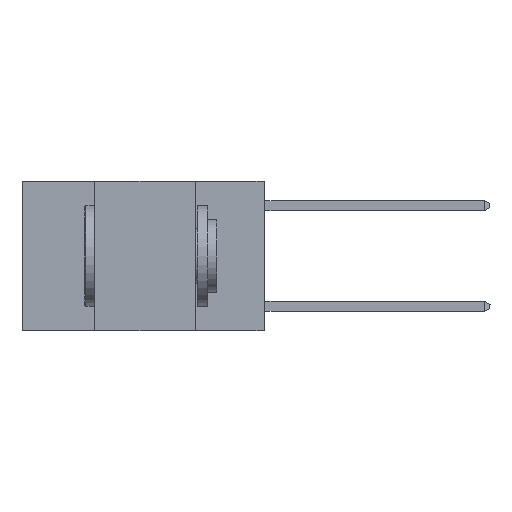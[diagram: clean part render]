
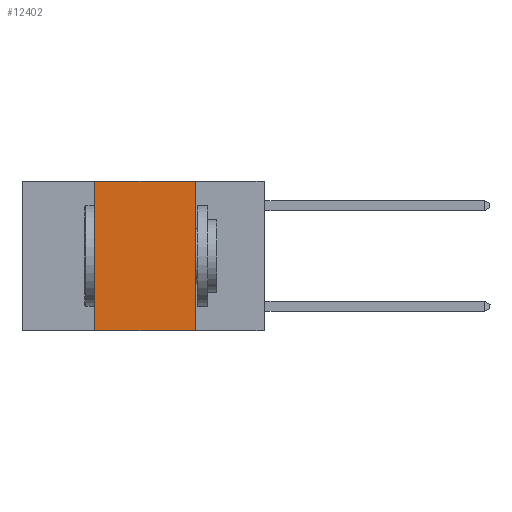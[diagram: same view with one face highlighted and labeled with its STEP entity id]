
A CAD part, left-side view. The second image highlights one B-rep face of the part: STEP entity #12402.
In plain terms, the highlighted planar face has unit normal (-1, 0, 0).
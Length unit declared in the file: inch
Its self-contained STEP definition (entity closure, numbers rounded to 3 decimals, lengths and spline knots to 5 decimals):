
#198 = PLANE ( 'NONE',  #18659 ) ;
#772 = VERTEX_POINT ( 'NONE', #2782 ) ;
#1118 = CARTESIAN_POINT ( 'NONE',  ( 0., 0.6, 0. ) ) ;
#1670 = DIRECTION ( 'NONE',  ( 1., 0., 0. ) ) ;
#1954 = DIRECTION ( 'NONE',  ( 0., 0., -1. ) ) ;
#2739 = VECTOR ( 'NONE', #11495, 39.37008 ) ;
#2782 = CARTESIAN_POINT ( 'NONE',  ( 0., 0.17, -0.37 ) ) ;
#4074 = CARTESIAN_POINT ( 'NONE',  ( 0., 0.42, 0. ) ) ;
#4597 = EDGE_CURVE ( 'NONE', #13266, #772, #5164, .T. ) ;
#5164 = LINE ( 'NONE', #9296, #12585 ) ;
#5683 = VERTEX_POINT ( 'NONE', #11790 ) ;
#5788 = FACE_OUTER_BOUND ( 'NONE', #7100, .T. ) ;
#6407 = CARTESIAN_POINT ( 'NONE',  ( 0., 0.17, 0. ) ) ;
#6696 = ORIENTED_EDGE ( 'NONE', *, *, #9893, .F. ) ;
#7100 = EDGE_LOOP ( 'NONE', ( #6696, #7524, #10214, #10619 ) ) ;
#7365 = VECTOR ( 'NONE', #12936, 39.37008 ) ;
#7524 = ORIENTED_EDGE ( 'NONE', *, *, #13277, .F. ) ;
#7794 = DIRECTION ( 'NONE',  ( 0., -1., 0. ) ) ;
#8744 = VERTEX_POINT ( 'NONE', #11118 ) ;
#8878 = LINE ( 'NONE', #6407, #16615 ) ;
#9296 = CARTESIAN_POINT ( 'NONE',  ( 0., 0.6, -0.37 ) ) ;
#9893 = EDGE_CURVE ( 'NONE', #8744, #772, #8878, .T. ) ;
#10214 = ORIENTED_EDGE ( 'NONE', *, *, #13925, .F. ) ;
#10565 = CARTESIAN_POINT ( 'NONE',  ( 0., 0.6, 0. ) ) ;
#10619 = ORIENTED_EDGE ( 'NONE', *, *, #4597, .T. ) ;
#11118 = CARTESIAN_POINT ( 'NONE',  ( 0., 0.17, 0. ) ) ;
#11429 = CARTESIAN_POINT ( 'NONE',  ( 0., 0.42, -0.37 ) ) ;
#11495 = DIRECTION ( 'NONE',  ( 0., -1., 0. ) ) ;
#11790 = CARTESIAN_POINT ( 'NONE',  ( 0., 0.42, 0. ) ) ;
#12046 = DIRECTION ( 'NONE',  ( 0., 0., -1. ) ) ;
#12402 = ADVANCED_FACE ( 'NONE', ( #5788 ), #198, .F. ) ;
#12585 = VECTOR ( 'NONE', #7794, 39.37008 ) ;
#12936 = DIRECTION ( 'NONE',  ( 0., 0., 1. ) ) ;
#13266 = VERTEX_POINT ( 'NONE', #11429 ) ;
#13277 = EDGE_CURVE ( 'NONE', #5683, #8744, #17845, .T. ) ;
#13925 = EDGE_CURVE ( 'NONE', #13266, #5683, #15142, .T. ) ;
#15142 = LINE ( 'NONE', #4074, #7365 ) ;
#16615 = VECTOR ( 'NONE', #1954, 39.37008 ) ;
#17845 = LINE ( 'NONE', #1118, #2739 ) ;
#18659 = AXIS2_PLACEMENT_3D ( 'NONE', #10565, #1670, #12046 ) ;
